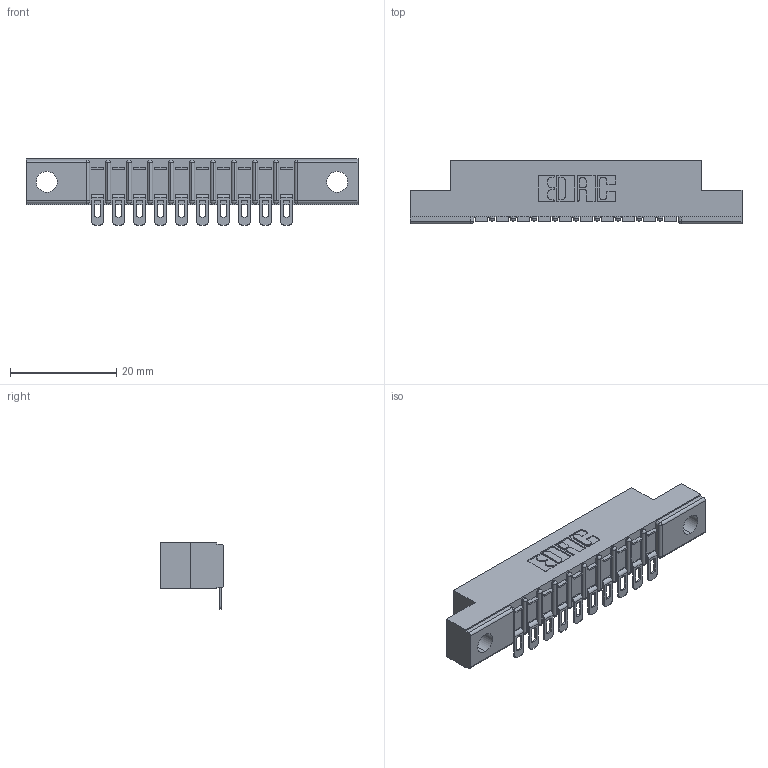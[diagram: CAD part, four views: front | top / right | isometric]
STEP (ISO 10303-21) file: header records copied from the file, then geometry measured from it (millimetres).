
FILE_DESCRIPTION (( 'STEP AP203' ), '1' );
FILE_NAME ('307-010-554-102.STEP', '2019-09-04T19:14:22', ( '' ), ( '' ), 'SwSTEP 2.0', 'SolidWorks 2016', '' );
FILE_SCHEMA (( 'CONFIG_CONTROL_DESIGN' ));
Length unit declared in the file: inch
Products named in the file (3): 307 Part_.128 Dia Mounting Holes; 307-290-002_554; 307-010-554-102
Assembly tree (11 placements, depth 2):
  307-010-554-102
    307 Part_.128 Dia Mounting Holes
    307-290-002_554  x10
Bounding box: 62.64 x 12.01 x 12.52 mm (x, y, z)
Volume: 4044.6 mm3; surface area: 6578.5 mm2
Topology: 11 solids, 11 shells, 939 faces, 2853 edges, 1870 vertices
Faces by surface type: plane 530, cylinder 387, sphere 22
Entity records: 13485 total; most frequent: CARTESIAN_POINT 2270, ORIENTED_EDGE 2260, DIRECTION 2226, EDGE_CURVE 1130, VECTOR 842, LINE 842, VERTEX_POINT 736, AXIS2_PLACEMENT_3D 692
